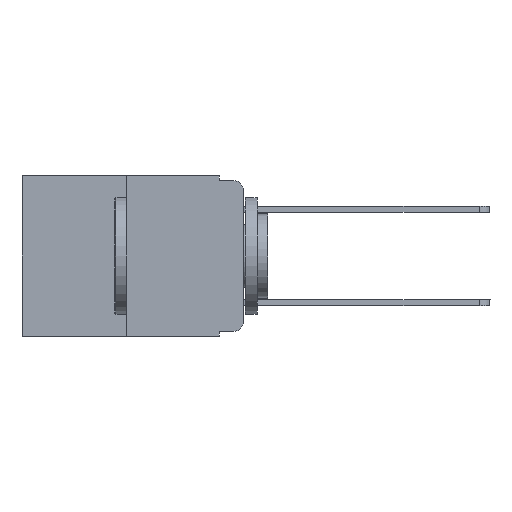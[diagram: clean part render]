
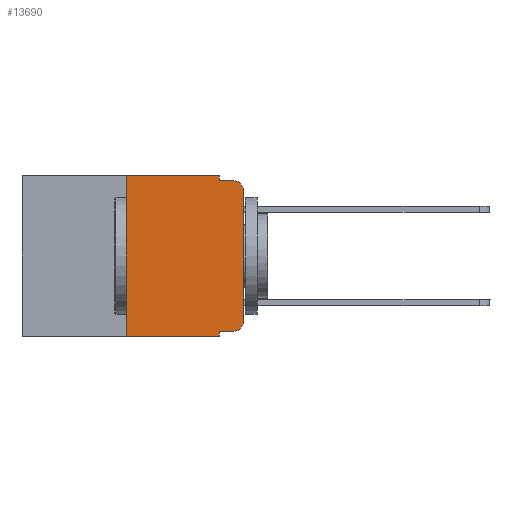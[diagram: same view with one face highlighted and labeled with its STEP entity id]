
A CAD part, left-side view. The second image highlights one B-rep face of the part: STEP entity #13690.
In plain terms, the highlighted planar face has unit normal (-1, 0, 0).
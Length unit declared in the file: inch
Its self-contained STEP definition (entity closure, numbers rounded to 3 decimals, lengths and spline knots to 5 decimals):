
#17 = CARTESIAN_POINT ( 'NONE',  ( 0., 0.25, 0. ) ) ;
#157 = DIRECTION ( 'NONE',  ( -1., 0., 0. ) ) ;
#290 = AXIS2_PLACEMENT_3D ( 'NONE', #7165, #15555, #10143 ) ;
#423 = CARTESIAN_POINT ( 'NONE',  ( 0., 0.02, -0.01 ) ) ;
#562 = VERTEX_POINT ( 'NONE', #423 ) ;
#1333 = CARTESIAN_POINT ( 'NONE',  ( 0., 0., 0. ) ) ;
#1417 = LINE ( 'NONE', #1333, #3020 ) ;
#1783 = DIRECTION ( 'NONE',  ( 0., -1., 0. ) ) ;
#2234 = ORIENTED_EDGE ( 'NONE', *, *, #6425, .F. ) ;
#2391 = CARTESIAN_POINT ( 'NONE',  ( 0., 0.051, -0.333 ) ) ;
#2622 = LINE ( 'NONE', #17, #8341 ) ;
#2744 = CARTESIAN_POINT ( 'NONE',  ( 0., 0.473, 0. ) ) ;
#2927 = VECTOR ( 'NONE', #9601, 39.37008 ) ;
#3020 = VECTOR ( 'NONE', #6827, 39.37008 ) ;
#4238 = VERTEX_POINT ( 'NONE', #16403 ) ;
#4656 = EDGE_CURVE ( 'NONE', #11043, #13692, #1417, .T. ) ;
#4680 = DIRECTION ( 'NONE',  ( 0., 0., -1. ) ) ;
#4725 = CARTESIAN_POINT ( 'NONE',  ( 0., 0.051, -0.01 ) ) ;
#4775 = CARTESIAN_POINT ( 'NONE',  ( 0., 0., -0.03 ) ) ;
#4893 = CARTESIAN_POINT ( 'NONE',  ( 0., 0.051, -0.343 ) ) ;
#4929 = VERTEX_POINT ( 'NONE', #2391 ) ;
#5386 = VECTOR ( 'NONE', #5757, 39.37008 ) ;
#5577 = EDGE_CURVE ( 'NONE', #10822, #9385, #2622, .T. ) ;
#5757 = DIRECTION ( 'NONE',  ( 0., -1., 0. ) ) ;
#5860 = ORIENTED_EDGE ( 'NONE', *, *, #6462, .T. ) ;
#5869 = CIRCLE ( 'NONE', #15917, 0.02 ) ;
#6425 = EDGE_CURVE ( 'NONE', #9385, #4238, #8354, .T. ) ;
#6462 = EDGE_CURVE ( 'NONE', #10822, #9482, #12327, .T. ) ;
#6827 = DIRECTION ( 'NONE',  ( 0., 0., 1. ) ) ;
#6850 = ORIENTED_EDGE ( 'NONE', *, *, #9629, .F. ) ;
#7066 = EDGE_CURVE ( 'NONE', #13692, #562, #16735, .T. ) ;
#7088 = CARTESIAN_POINT ( 'NONE',  ( 0., 0.051, -0.333 ) ) ;
#7165 = CARTESIAN_POINT ( 'NONE',  ( 0., 0.473, 0. ) ) ;
#7672 = CARTESIAN_POINT ( 'NONE',  ( 0., 0.25, -0.343 ) ) ;
#7815 = AXIS2_PLACEMENT_3D ( 'NONE', #15538, #12658, #4680 ) ;
#8341 = VECTOR ( 'NONE', #9497, 39.37008 ) ;
#8354 = LINE ( 'NONE', #2744, #13556 ) ;
#8363 = CARTESIAN_POINT ( 'NONE',  ( 0., 0., -0.313 ) ) ;
#8880 = EDGE_CURVE ( 'NONE', #4238, #15713, #9682, .T. ) ;
#8883 = ORIENTED_EDGE ( 'NONE', *, *, #9833, .T. ) ;
#9295 = ORIENTED_EDGE ( 'NONE', *, *, #17226, .F. ) ;
#9385 = VERTEX_POINT ( 'NONE', #12615 ) ;
#9432 = DIRECTION ( 'NONE',  ( 0., -1., 0. ) ) ;
#9482 = VERTEX_POINT ( 'NONE', #4893 ) ;
#9497 = DIRECTION ( 'NONE',  ( 0., 0., 1. ) ) ;
#9601 = DIRECTION ( 'NONE',  ( 0., 0., -1. ) ) ;
#9629 = EDGE_CURVE ( 'NONE', #4929, #9482, #13062, .T. ) ;
#9682 = LINE ( 'NONE', #12663, #2927 ) ;
#9833 = EDGE_CURVE ( 'NONE', #9935, #11043, #5869, .T. ) ;
#9888 = DIRECTION ( 'NONE',  ( 0., 0., -1. ) ) ;
#9935 = VERTEX_POINT ( 'NONE', #15382 ) ;
#10024 = ORIENTED_EDGE ( 'NONE', *, *, #5577, .F. ) ;
#10050 = ORIENTED_EDGE ( 'NONE', *, *, #11061, .T. ) ;
#10143 = DIRECTION ( 'NONE',  ( 0., 0., -1. ) ) ;
#10705 = DIRECTION ( 'NONE',  ( 0., 0., -1. ) ) ;
#10822 = VERTEX_POINT ( 'NONE', #7672 ) ;
#11019 = ORIENTED_EDGE ( 'NONE', *, *, #4656, .T. ) ;
#11043 = VERTEX_POINT ( 'NONE', #8363 ) ;
#11061 = EDGE_CURVE ( 'NONE', #4929, #9935, #14136, .T. ) ;
#11240 = VECTOR ( 'NONE', #9432, 39.37008 ) ;
#11418 = CARTESIAN_POINT ( 'NONE',  ( 0., 0.02, -0.313 ) ) ;
#11839 = VECTOR ( 'NONE', #1783, 39.37008 ) ;
#12013 = CARTESIAN_POINT ( 'NONE',  ( 0., 0.051, -0.01 ) ) ;
#12239 = CARTESIAN_POINT ( 'NONE',  ( 0., 0.473, -0.343 ) ) ;
#12327 = LINE ( 'NONE', #12239, #11240 ) ;
#12414 = DIRECTION ( 'NONE',  ( 0., -1., 0. ) ) ;
#12615 = CARTESIAN_POINT ( 'NONE',  ( 0., 0.25, 0. ) ) ;
#12658 = DIRECTION ( 'NONE',  ( -1., 0., 0. ) ) ;
#12663 = CARTESIAN_POINT ( 'NONE',  ( 0., 0.051, 0. ) ) ;
#12766 = PLANE ( 'NONE',  #290 ) ;
#13062 = LINE ( 'NONE', #16284, #17344 ) ;
#13556 = VECTOR ( 'NONE', #12414, 39.37008 ) ;
#13690 = ADVANCED_FACE ( 'NONE', ( #15643 ), #12766, .F. ) ;
#13692 = VERTEX_POINT ( 'NONE', #4775 ) ;
#14136 = LINE ( 'NONE', #7088, #5386 ) ;
#15382 = CARTESIAN_POINT ( 'NONE',  ( 0., 0.02, -0.333 ) ) ;
#15538 = CARTESIAN_POINT ( 'NONE',  ( 0., 0.02, -0.03 ) ) ;
#15555 = DIRECTION ( 'NONE',  ( 1., 0., 0. ) ) ;
#15582 = LINE ( 'NONE', #4725, #11839 ) ;
#15643 = FACE_OUTER_BOUND ( 'NONE', #17688, .T. ) ;
#15713 = VERTEX_POINT ( 'NONE', #12013 ) ;
#15898 = ORIENTED_EDGE ( 'NONE', *, *, #7066, .T. ) ;
#15917 = AXIS2_PLACEMENT_3D ( 'NONE', #11418, #157, #9888 ) ;
#16284 = CARTESIAN_POINT ( 'NONE',  ( 0., 0.051, 0. ) ) ;
#16403 = CARTESIAN_POINT ( 'NONE',  ( 0., 0.051, 0. ) ) ;
#16735 = CIRCLE ( 'NONE', #7815, 0.02 ) ;
#17089 = ORIENTED_EDGE ( 'NONE', *, *, #8880, .F. ) ;
#17226 = EDGE_CURVE ( 'NONE', #15713, #562, #15582, .T. ) ;
#17344 = VECTOR ( 'NONE', #10705, 39.37008 ) ;
#17688 = EDGE_LOOP ( 'NONE', ( #11019, #15898, #9295, #17089, #2234, #10024, #5860, #6850, #10050, #8883 ) ) ;
